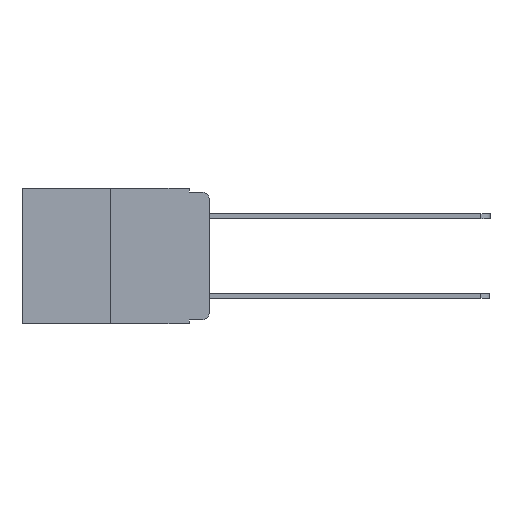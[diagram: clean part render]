
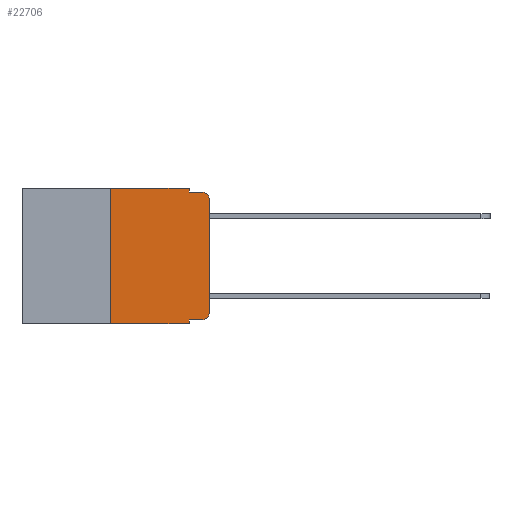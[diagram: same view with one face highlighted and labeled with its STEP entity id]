
A CAD part, left-side view. The second image highlights one B-rep face of the part: STEP entity #22706.
In plain terms, the highlighted planar face has unit normal (-1, 0, 0).
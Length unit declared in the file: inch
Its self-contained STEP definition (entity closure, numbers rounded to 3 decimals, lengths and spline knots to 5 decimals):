
#314 = CARTESIAN_POINT ( 'NONE',  ( 0., 0.051, -0.333 ) ) ;
#1011 = EDGE_CURVE ( 'NONE', #9340, #18478, #19040, .T. ) ;
#1498 = DIRECTION ( 'NONE',  ( -1., 0., 0. ) ) ;
#1729 = DIRECTION ( 'NONE',  ( 0., -1., 0. ) ) ;
#1830 = AXIS2_PLACEMENT_3D ( 'NONE', #12430, #1498, #14226 ) ;
#1993 = CARTESIAN_POINT ( 'NONE',  ( 0., 0.051, 0. ) ) ;
#2076 = ORIENTED_EDGE ( 'NONE', *, *, #1011, .F. ) ;
#2229 = VECTOR ( 'NONE', #16408, 39.37008 ) ;
#2464 = VERTEX_POINT ( 'NONE', #21689 ) ;
#2705 = CARTESIAN_POINT ( 'NONE',  ( 0., 0., 0. ) ) ;
#2758 = EDGE_CURVE ( 'NONE', #3044, #5762, #9140, .T. ) ;
#2819 = LINE ( 'NONE', #1993, #2229 ) ;
#3044 = VERTEX_POINT ( 'NONE', #314 ) ;
#3097 = CARTESIAN_POINT ( 'NONE',  ( 0., 0.473, 0. ) ) ;
#3222 = DIRECTION ( 'NONE',  ( 0., 0., 1. ) ) ;
#3432 = ORIENTED_EDGE ( 'NONE', *, *, #14434, .F. ) ;
#3451 = VECTOR ( 'NONE', #15695, 39.37008 ) ;
#3666 = DIRECTION ( 'NONE',  ( -1., 0., 0. ) ) ;
#4055 = ORIENTED_EDGE ( 'NONE', *, *, #15174, .T. ) ;
#4364 = VECTOR ( 'NONE', #18632, 39.37008 ) ;
#4423 = ORIENTED_EDGE ( 'NONE', *, *, #19944, .F. ) ;
#4577 = DIRECTION ( 'NONE',  ( 0., 0., 1. ) ) ;
#4595 = AXIS2_PLACEMENT_3D ( 'NONE', #17603, #21162, #10754 ) ;
#5762 = VERTEX_POINT ( 'NONE', #10065 ) ;
#5901 = VECTOR ( 'NONE', #11839, 39.37008 ) ;
#6689 = CIRCLE ( 'NONE', #13149, 0.02 ) ;
#6949 = DIRECTION ( 'NONE',  ( 0., -1., 0. ) ) ;
#7004 = ORIENTED_EDGE ( 'NONE', *, *, #13536, .F. ) ;
#7595 = CARTESIAN_POINT ( 'NONE',  ( 0., 0.051, -0.333 ) ) ;
#8386 = CARTESIAN_POINT ( 'NONE',  ( 0., 0., -0.313 ) ) ;
#8591 = LINE ( 'NONE', #3097, #3451 ) ;
#8966 = CARTESIAN_POINT ( 'NONE',  ( 0., 0., -0.03 ) ) ;
#9140 = LINE ( 'NONE', #7595, #13313 ) ;
#9227 = VECTOR ( 'NONE', #3222, 39.37008 ) ;
#9340 = VERTEX_POINT ( 'NONE', #16478 ) ;
#9815 = LINE ( 'NONE', #16882, #4364 ) ;
#9964 = VECTOR ( 'NONE', #4577, 39.37008 ) ;
#10065 = CARTESIAN_POINT ( 'NONE',  ( 0., 0.02, -0.333 ) ) ;
#10071 = CARTESIAN_POINT ( 'NONE',  ( 0., 0.473, -0.343 ) ) ;
#10138 = EDGE_CURVE ( 'NONE', #3044, #21505, #9815, .T. ) ;
#10261 = VERTEX_POINT ( 'NONE', #22371 ) ;
#10389 = VERTEX_POINT ( 'NONE', #14104 ) ;
#10754 = DIRECTION ( 'NONE',  ( 0., 0., -1. ) ) ;
#11273 = ORIENTED_EDGE ( 'NONE', *, *, #10138, .F. ) ;
#11839 = DIRECTION ( 'NONE',  ( 0., -1., 0. ) ) ;
#12430 = CARTESIAN_POINT ( 'NONE',  ( 0., 0.02, -0.313 ) ) ;
#12610 = CARTESIAN_POINT ( 'NONE',  ( 0., 0.02, -0.01 ) ) ;
#13149 = AXIS2_PLACEMENT_3D ( 'NONE', #14499, #3666, #16227 ) ;
#13313 = VECTOR ( 'NONE', #1729, 39.37008 ) ;
#13346 = CARTESIAN_POINT ( 'NONE',  ( 0., 0.051, -0.01 ) ) ;
#13536 = EDGE_CURVE ( 'NONE', #10261, #10389, #8591, .T. ) ;
#14104 = CARTESIAN_POINT ( 'NONE',  ( 0., 0.051, 0. ) ) ;
#14226 = DIRECTION ( 'NONE',  ( 0., 0., -1. ) ) ;
#14434 = EDGE_CURVE ( 'NONE', #10389, #9340, #2819, .T. ) ;
#14442 = VECTOR ( 'NONE', #6949, 39.37008 ) ;
#14499 = CARTESIAN_POINT ( 'NONE',  ( 0., 0.02, -0.03 ) ) ;
#15134 = ORIENTED_EDGE ( 'NONE', *, *, #2758, .T. ) ;
#15174 = EDGE_CURVE ( 'NONE', #21703, #19438, #15221, .T. ) ;
#15221 = LINE ( 'NONE', #2705, #9964 ) ;
#15434 = LINE ( 'NONE', #10071, #5901 ) ;
#15695 = DIRECTION ( 'NONE',  ( 0., -1., 0. ) ) ;
#16227 = DIRECTION ( 'NONE',  ( 0., 0., -1. ) ) ;
#16408 = DIRECTION ( 'NONE',  ( 0., 0., -1. ) ) ;
#16478 = CARTESIAN_POINT ( 'NONE',  ( 0., 0.051, -0.01 ) ) ;
#16882 = CARTESIAN_POINT ( 'NONE',  ( 0., 0.051, 0. ) ) ;
#17150 = EDGE_CURVE ( 'NONE', #5762, #21703, #22890, .T. ) ;
#17603 = CARTESIAN_POINT ( 'NONE',  ( 0., 0.473, 0. ) ) ;
#17870 = EDGE_CURVE ( 'NONE', #19438, #18478, #6689, .T. ) ;
#18391 = ORIENTED_EDGE ( 'NONE', *, *, #17870, .T. ) ;
#18478 = VERTEX_POINT ( 'NONE', #12610 ) ;
#18632 = DIRECTION ( 'NONE',  ( 0., 0., -1. ) ) ;
#18674 = EDGE_LOOP ( 'NONE', ( #4055, #18391, #2076, #3432, #7004, #4423, #21150, #11273, #15134, #18896 ) ) ;
#18896 = ORIENTED_EDGE ( 'NONE', *, *, #17150, .T. ) ;
#19040 = LINE ( 'NONE', #13346, #14442 ) ;
#19438 = VERTEX_POINT ( 'NONE', #8966 ) ;
#19944 = EDGE_CURVE ( 'NONE', #2464, #10261, #20175, .T. ) ;
#20175 = LINE ( 'NONE', #22633, #9227 ) ;
#20274 = FACE_OUTER_BOUND ( 'NONE', #18674, .T. ) ;
#21150 = ORIENTED_EDGE ( 'NONE', *, *, #22465, .T. ) ;
#21162 = DIRECTION ( 'NONE',  ( 1., 0., 0. ) ) ;
#21505 = VERTEX_POINT ( 'NONE', #21750 ) ;
#21689 = CARTESIAN_POINT ( 'NONE',  ( 0., 0.25, -0.343 ) ) ;
#21703 = VERTEX_POINT ( 'NONE', #8386 ) ;
#21750 = CARTESIAN_POINT ( 'NONE',  ( 0., 0.051, -0.343 ) ) ;
#22371 = CARTESIAN_POINT ( 'NONE',  ( 0., 0.25, 0. ) ) ;
#22465 = EDGE_CURVE ( 'NONE', #2464, #21505, #15434, .T. ) ;
#22633 = CARTESIAN_POINT ( 'NONE',  ( 0., 0.25, 0. ) ) ;
#22706 = ADVANCED_FACE ( 'NONE', ( #20274 ), #22805, .F. ) ;
#22805 = PLANE ( 'NONE',  #4595 ) ;
#22890 = CIRCLE ( 'NONE', #1830, 0.02 ) ;
